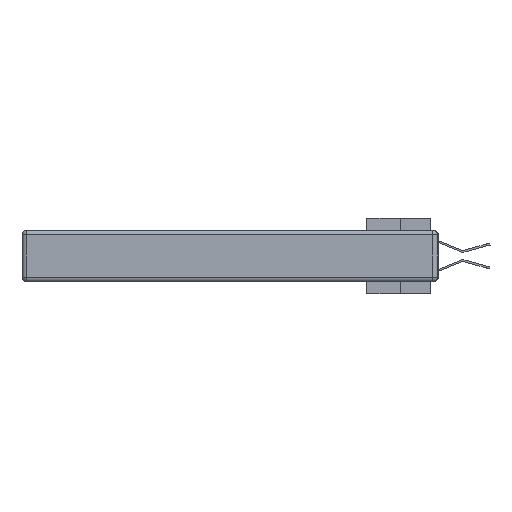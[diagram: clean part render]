
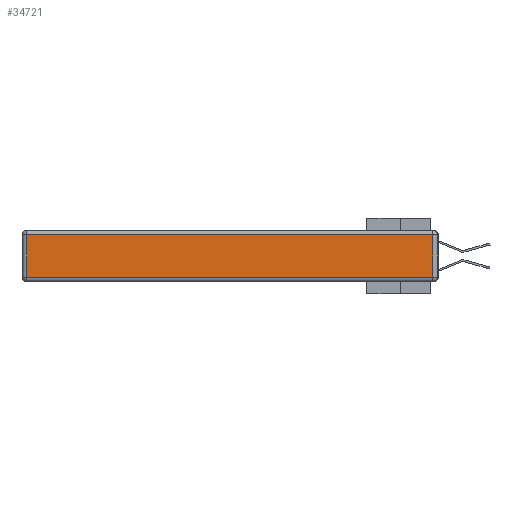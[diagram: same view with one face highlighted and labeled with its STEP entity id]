
A CAD part, left-side view. The second image highlights one B-rep face of the part: STEP entity #34721.
In plain terms, the highlighted planar face has unit normal (-1, 0, 0).
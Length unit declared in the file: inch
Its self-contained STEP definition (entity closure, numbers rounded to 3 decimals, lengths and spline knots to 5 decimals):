
#1290 = DIRECTION ( 'NONE',  ( 0., -1., 0. ) ) ;
#1861 = FACE_OUTER_BOUND ( 'NONE', #28747, .T. ) ;
#2356 = CARTESIAN_POINT ( 'NONE',  ( 0., 2.72, -0.343 ) ) ;
#2678 = ORIENTED_EDGE ( 'NONE', *, *, #3575, .T. ) ;
#3436 = CARTESIAN_POINT ( 'NONE',  ( 0., 0.03, -0.03 ) ) ;
#3491 = VECTOR ( 'NONE', #35368, 39.37008 ) ;
#3575 = EDGE_CURVE ( 'NONE', #22223, #19175, #29955, .T. ) ;
#4357 = DIRECTION ( 'NONE',  ( 0., 0., 1. ) ) ;
#4573 = DIRECTION ( 'NONE',  ( -1., 0., 0. ) ) ;
#4928 = LINE ( 'NONE', #13408, #13117 ) ;
#7647 = CARTESIAN_POINT ( 'NONE',  ( 0., 0., -0.343 ) ) ;
#9416 = LINE ( 'NONE', #18067, #17600 ) ;
#10797 = VECTOR ( 'NONE', #1290, 39.37008 ) ;
#12194 = CARTESIAN_POINT ( 'NONE',  ( 0., 2.72, -0.03 ) ) ;
#13073 = ORIENTED_EDGE ( 'NONE', *, *, #14570, .T. ) ;
#13117 = VECTOR ( 'NONE', #15930, 39.37008 ) ;
#13408 = CARTESIAN_POINT ( 'NONE',  ( 0., 2.75, -0.03 ) ) ;
#14570 = EDGE_CURVE ( 'NONE', #20391, #24627, #9416, .T. ) ;
#14639 = LINE ( 'NONE', #22767, #10797 ) ;
#15112 = CARTESIAN_POINT ( 'NONE',  ( 0., 2.72, -0.313 ) ) ;
#15120 = CARTESIAN_POINT ( 'NONE',  ( 0., 0.03, -0.313 ) ) ;
#15579 = PLANE ( 'NONE',  #20154 ) ;
#15744 = DIRECTION ( 'NONE',  ( 0., 0., 1. ) ) ;
#15930 = DIRECTION ( 'NONE',  ( 0., 1., 0. ) ) ;
#17600 = VECTOR ( 'NONE', #4357, 39.37008 ) ;
#18067 = CARTESIAN_POINT ( 'NONE',  ( 0., 0.03, -0.343 ) ) ;
#19175 = VERTEX_POINT ( 'NONE', #15112 ) ;
#20154 = AXIS2_PLACEMENT_3D ( 'NONE', #7647, #4573, #15744 ) ;
#20391 = VERTEX_POINT ( 'NONE', #15120 ) ;
#21250 = ORIENTED_EDGE ( 'NONE', *, *, #22799, .T. ) ;
#22223 = VERTEX_POINT ( 'NONE', #12194 ) ;
#22767 = CARTESIAN_POINT ( 'NONE',  ( 0., 0., -0.313 ) ) ;
#22799 = EDGE_CURVE ( 'NONE', #24627, #22223, #4928, .T. ) ;
#24627 = VERTEX_POINT ( 'NONE', #3436 ) ;
#28747 = EDGE_LOOP ( 'NONE', ( #31350, #13073, #21250, #2678 ) ) ;
#29955 = LINE ( 'NONE', #2356, #3491 ) ;
#31350 = ORIENTED_EDGE ( 'NONE', *, *, #32663, .T. ) ;
#32663 = EDGE_CURVE ( 'NONE', #19175, #20391, #14639, .T. ) ;
#34721 = ADVANCED_FACE ( 'NONE', ( #1861 ), #15579, .T. ) ;
#35368 = DIRECTION ( 'NONE',  ( 0., 0., -1. ) ) ;
